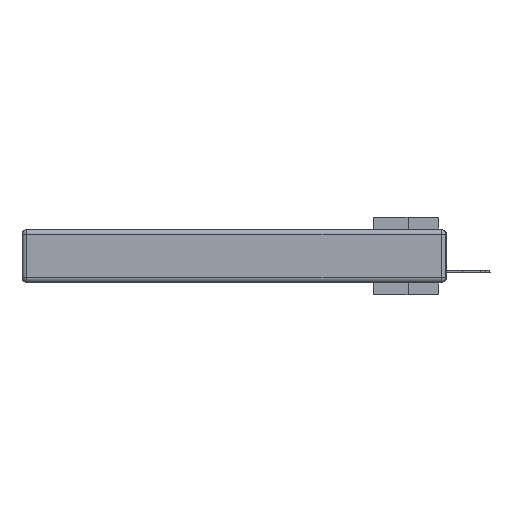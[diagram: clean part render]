
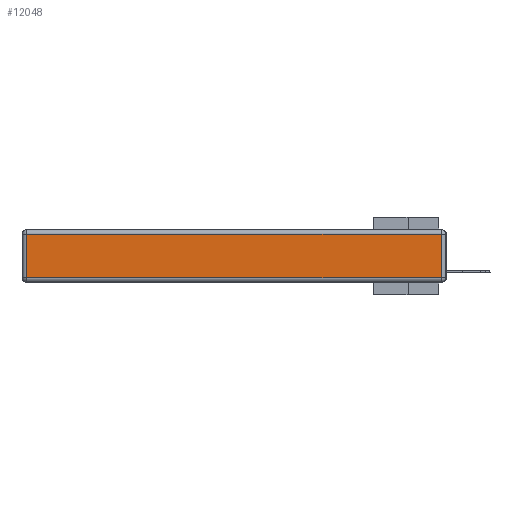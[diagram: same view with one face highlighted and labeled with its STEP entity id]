
A CAD part, left-side view. The second image highlights one B-rep face of the part: STEP entity #12048.
In plain terms, the highlighted planar face has unit normal (-1, 0, 0).
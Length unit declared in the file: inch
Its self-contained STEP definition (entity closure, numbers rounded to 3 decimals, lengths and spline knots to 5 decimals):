
#111 = EDGE_CURVE ( 'NONE', #29068, #16472, #26544, .T. ) ;
#368 = ORIENTED_EDGE ( 'NONE', *, *, #13773, .T. ) ;
#640 = AXIS2_PLACEMENT_3D ( 'NONE', #20044, #22506, #8236 ) ;
#1874 = FACE_OUTER_BOUND ( 'NONE', #21776, .T. ) ;
#2331 = VERTEX_POINT ( 'NONE', #29939 ) ;
#2727 = LINE ( 'NONE', #21105, #14220 ) ;
#2754 = DIRECTION ( 'NONE',  ( 0., -1., 0. ) ) ;
#3267 = PLANE ( 'NONE',  #640 ) ;
#6454 = DIRECTION ( 'NONE',  ( 0., 1., 0. ) ) ;
#7413 = LINE ( 'NONE', #28919, #12647 ) ;
#8236 = DIRECTION ( 'NONE',  ( 0., 0., 1. ) ) ;
#9653 = CARTESIAN_POINT ( 'NONE',  ( 0., 0.03, -0.343 ) ) ;
#10263 = VECTOR ( 'NONE', #6454, 39.37008 ) ;
#10683 = ORIENTED_EDGE ( 'NONE', *, *, #111, .T. ) ;
#11775 = DIRECTION ( 'NONE',  ( 0., 0., 1. ) ) ;
#12048 = ADVANCED_FACE ( 'NONE', ( #1874 ), #3267, .T. ) ;
#12647 = VECTOR ( 'NONE', #2754, 39.37008 ) ;
#13497 = CARTESIAN_POINT ( 'NONE',  ( 0., 0.03, -0.313 ) ) ;
#13773 = EDGE_CURVE ( 'NONE', #16432, #29068, #26877, .T. ) ;
#14220 = VECTOR ( 'NONE', #16427, 39.37008 ) ;
#16427 = DIRECTION ( 'NONE',  ( 0., 0., -1. ) ) ;
#16432 = VERTEX_POINT ( 'NONE', #13497 ) ;
#16472 = VERTEX_POINT ( 'NONE', #22770 ) ;
#17236 = ORIENTED_EDGE ( 'NONE', *, *, #19716, .T. ) ;
#19716 = EDGE_CURVE ( 'NONE', #2331, #16432, #7413, .T. ) ;
#20044 = CARTESIAN_POINT ( 'NONE',  ( 0., 0., -0.343 ) ) ;
#21105 = CARTESIAN_POINT ( 'NONE',  ( 0., 2.72, -0.343 ) ) ;
#21776 = EDGE_LOOP ( 'NONE', ( #17236, #368, #10683, #25911 ) ) ;
#22428 = VECTOR ( 'NONE', #11775, 39.37008 ) ;
#22506 = DIRECTION ( 'NONE',  ( -1., 0., 0. ) ) ;
#22770 = CARTESIAN_POINT ( 'NONE',  ( 0., 2.72, -0.03 ) ) ;
#22798 = CARTESIAN_POINT ( 'NONE',  ( 0., 2.75, -0.03 ) ) ;
#25650 = EDGE_CURVE ( 'NONE', #16472, #2331, #2727, .T. ) ;
#25911 = ORIENTED_EDGE ( 'NONE', *, *, #25650, .T. ) ;
#26035 = CARTESIAN_POINT ( 'NONE',  ( 0., 0.03, -0.03 ) ) ;
#26544 = LINE ( 'NONE', #22798, #10263 ) ;
#26877 = LINE ( 'NONE', #9653, #22428 ) ;
#28919 = CARTESIAN_POINT ( 'NONE',  ( 0., 0., -0.313 ) ) ;
#29068 = VERTEX_POINT ( 'NONE', #26035 ) ;
#29939 = CARTESIAN_POINT ( 'NONE',  ( 0., 2.72, -0.313 ) ) ;
